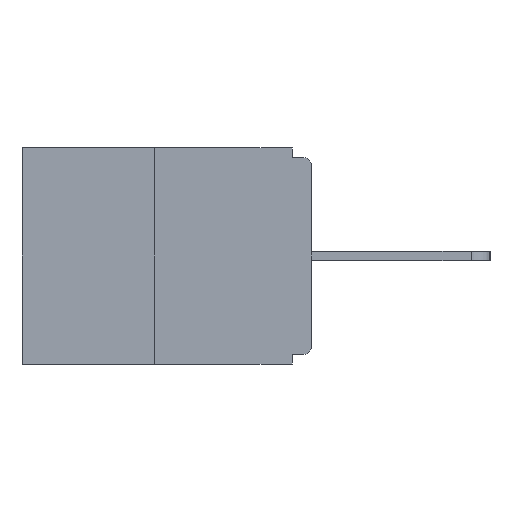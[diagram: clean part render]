
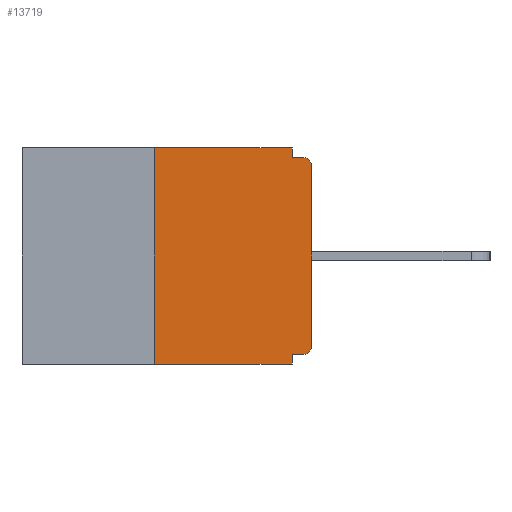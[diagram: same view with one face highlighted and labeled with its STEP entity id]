
A CAD part, left-side view. The second image highlights one B-rep face of the part: STEP entity #13719.
In plain terms, the highlighted planar face has unit normal (-1, 0, 0).
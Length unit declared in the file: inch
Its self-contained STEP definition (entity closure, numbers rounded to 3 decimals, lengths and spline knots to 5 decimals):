
#1536 = LINE ( 'NONE', #14418, #23593 ) ;
#2735 = CARTESIAN_POINT ( 'NONE',  ( 0., 0.015, -0.03 ) ) ;
#2765 = ORIENTED_EDGE ( 'NONE', *, *, #23916, .F. ) ;
#2894 = VECTOR ( 'NONE', #8748, 39.37008 ) ;
#2903 = CARTESIAN_POINT ( 'NONE',  ( 0., 0.031, 0. ) ) ;
#2975 = EDGE_CURVE ( 'NONE', #25251, #22243, #1536, .T. ) ;
#3259 = VERTEX_POINT ( 'NONE', #11903 ) ;
#3412 = DIRECTION ( 'NONE',  ( 0., -1., 0. ) ) ;
#3716 = VERTEX_POINT ( 'NONE', #16053 ) ;
#3729 = CARTESIAN_POINT ( 'NONE',  ( 0., 0.25, -0.343 ) ) ;
#3926 = EDGE_CURVE ( 'NONE', #25251, #16651, #4486, .T. ) ;
#3982 = EDGE_CURVE ( 'NONE', #3259, #4383, #11119, .T. ) ;
#4155 = VECTOR ( 'NONE', #15717, 39.37008 ) ;
#4165 = CARTESIAN_POINT ( 'NONE',  ( 0., 0.031, -0.328 ) ) ;
#4383 = VERTEX_POINT ( 'NONE', #17051 ) ;
#4486 = LINE ( 'NONE', #6219, #23531 ) ;
#4764 = FACE_OUTER_BOUND ( 'NONE', #25935, .T. ) ;
#5546 = VECTOR ( 'NONE', #15260, 39.37008 ) ;
#6219 = CARTESIAN_POINT ( 'NONE',  ( 0., 0.25, 0. ) ) ;
#6440 = EDGE_CURVE ( 'NONE', #3716, #19250, #13820, .T. ) ;
#6446 = CARTESIAN_POINT ( 'NONE',  ( 0., 0., -0.328 ) ) ;
#6564 = VERTEX_POINT ( 'NONE', #10122 ) ;
#6968 = CARTESIAN_POINT ( 'NONE',  ( 0., 0.015, -0.313 ) ) ;
#7187 = ORIENTED_EDGE ( 'NONE', *, *, #3982, .T. ) ;
#8748 = DIRECTION ( 'NONE',  ( 0., 1., 0. ) ) ;
#8795 = VECTOR ( 'NONE', #24392, 39.37008 ) ;
#9087 = DIRECTION ( 'NONE',  ( 0., 0., -1. ) ) ;
#9292 = CARTESIAN_POINT ( 'NONE',  ( 0., 0.031, -0.343 ) ) ;
#10122 = CARTESIAN_POINT ( 'NONE',  ( 0., 0.031, 0. ) ) ;
#10503 = CARTESIAN_POINT ( 'NONE',  ( 0., 0., -0.03 ) ) ;
#10824 = DIRECTION ( 'NONE',  ( -1., 0., 0. ) ) ;
#11030 = ORIENTED_EDGE ( 'NONE', *, *, #6440, .F. ) ;
#11119 = CIRCLE ( 'NONE', #25484, 0.015 ) ;
#11772 = CARTESIAN_POINT ( 'NONE',  ( 0., 0.46, 0. ) ) ;
#11802 = CARTESIAN_POINT ( 'NONE',  ( 0., 0.46, 0. ) ) ;
#11903 = CARTESIAN_POINT ( 'NONE',  ( 0., 0.015, -0.328 ) ) ;
#12140 = LINE ( 'NONE', #11772, #8795 ) ;
#13070 = ORIENTED_EDGE ( 'NONE', *, *, #24189, .F. ) ;
#13719 = ADVANCED_FACE ( 'NONE', ( #4764 ), #18049, .F. ) ;
#13820 = LINE ( 'NONE', #20397, #15471 ) ;
#14418 = CARTESIAN_POINT ( 'NONE',  ( 0., 0.46, -0.343 ) ) ;
#14437 = LINE ( 'NONE', #2903, #4155 ) ;
#15150 = LINE ( 'NONE', #9292, #18096 ) ;
#15260 = DIRECTION ( 'NONE',  ( 0., 0., 1. ) ) ;
#15438 = EDGE_CURVE ( 'NONE', #25646, #19250, #15871, .T. ) ;
#15471 = VECTOR ( 'NONE', #3412, 39.37008 ) ;
#15717 = DIRECTION ( 'NONE',  ( 0., 0., -1. ) ) ;
#15871 = CIRCLE ( 'NONE', #26584, 0.015 ) ;
#15875 = CARTESIAN_POINT ( 'NONE',  ( 0., 0.031, -0.343 ) ) ;
#15991 = DIRECTION ( 'NONE',  ( 0., 0., -1. ) ) ;
#16053 = CARTESIAN_POINT ( 'NONE',  ( 0., 0.031, -0.015 ) ) ;
#16651 = VERTEX_POINT ( 'NONE', #25836 ) ;
#16895 = AXIS2_PLACEMENT_3D ( 'NONE', #11802, #26796, #15991 ) ;
#17051 = CARTESIAN_POINT ( 'NONE',  ( 0., 0., -0.313 ) ) ;
#17340 = ORIENTED_EDGE ( 'NONE', *, *, #24291, .F. ) ;
#17511 = ORIENTED_EDGE ( 'NONE', *, *, #2975, .T. ) ;
#17628 = DIRECTION ( 'NONE',  ( 0., 0., -1. ) ) ;
#17862 = LINE ( 'NONE', #6446, #2894 ) ;
#17984 = EDGE_CURVE ( 'NONE', #4383, #25646, #26886, .T. ) ;
#18040 = EDGE_CURVE ( 'NONE', #3259, #24995, #17862, .T. ) ;
#18049 = PLANE ( 'NONE',  #16895 ) ;
#18096 = VECTOR ( 'NONE', #9087, 39.37008 ) ;
#18450 = ORIENTED_EDGE ( 'NONE', *, *, #3926, .F. ) ;
#19250 = VERTEX_POINT ( 'NONE', #21335 ) ;
#20397 = CARTESIAN_POINT ( 'NONE',  ( 0., 0., -0.015 ) ) ;
#21231 = ORIENTED_EDGE ( 'NONE', *, *, #15438, .T. ) ;
#21233 = DIRECTION ( 'NONE',  ( 0., 0., 1. ) ) ;
#21335 = CARTESIAN_POINT ( 'NONE',  ( 0., 0.015, -0.015 ) ) ;
#21374 = CARTESIAN_POINT ( 'NONE',  ( 0., 0., 0. ) ) ;
#21605 = DIRECTION ( 'NONE',  ( -1., 0., 0. ) ) ;
#21865 = DIRECTION ( 'NONE',  ( 0., 0., -1. ) ) ;
#22243 = VERTEX_POINT ( 'NONE', #15875 ) ;
#23444 = ORIENTED_EDGE ( 'NONE', *, *, #18040, .F. ) ;
#23531 = VECTOR ( 'NONE', #21233, 39.37008 ) ;
#23593 = VECTOR ( 'NONE', #27508, 39.37008 ) ;
#23916 = EDGE_CURVE ( 'NONE', #6564, #3716, #14437, .T. ) ;
#24189 = EDGE_CURVE ( 'NONE', #24995, #22243, #15150, .T. ) ;
#24291 = EDGE_CURVE ( 'NONE', #16651, #6564, #12140, .T. ) ;
#24392 = DIRECTION ( 'NONE',  ( 0., -1., 0. ) ) ;
#24995 = VERTEX_POINT ( 'NONE', #4165 ) ;
#25251 = VERTEX_POINT ( 'NONE', #3729 ) ;
#25484 = AXIS2_PLACEMENT_3D ( 'NONE', #6968, #21605, #21865 ) ;
#25646 = VERTEX_POINT ( 'NONE', #10503 ) ;
#25836 = CARTESIAN_POINT ( 'NONE',  ( 0., 0.25, 0. ) ) ;
#25935 = EDGE_LOOP ( 'NONE', ( #17340, #18450, #17511, #13070, #23444, #7187, #26734, #21231, #11030, #2765 ) ) ;
#26584 = AXIS2_PLACEMENT_3D ( 'NONE', #2735, #10824, #17628 ) ;
#26734 = ORIENTED_EDGE ( 'NONE', *, *, #17984, .T. ) ;
#26796 = DIRECTION ( 'NONE',  ( 1., 0., 0. ) ) ;
#26886 = LINE ( 'NONE', #21374, #5546 ) ;
#27508 = DIRECTION ( 'NONE',  ( 0., -1., 0. ) ) ;
